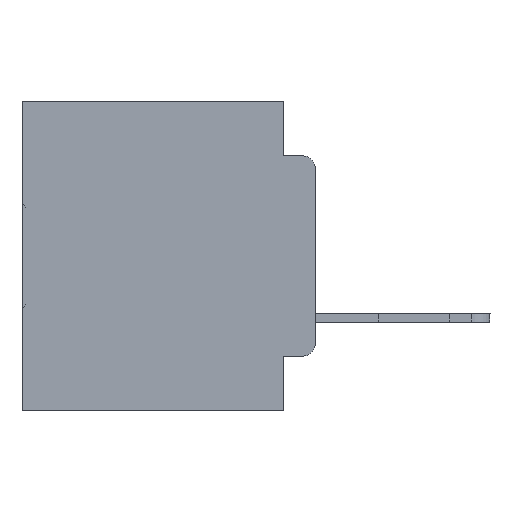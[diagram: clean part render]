
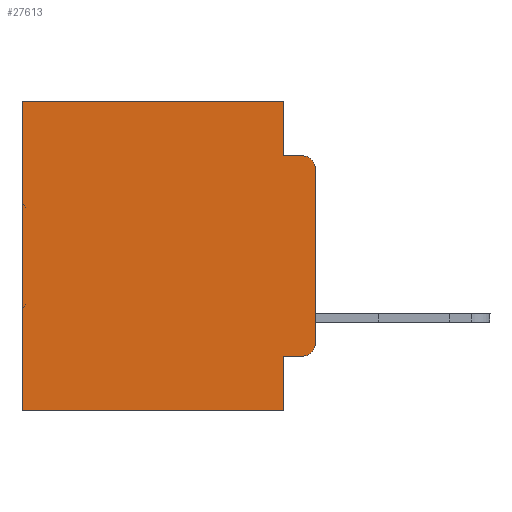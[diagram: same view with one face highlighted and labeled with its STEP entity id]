
A CAD part, left-side view. The second image highlights one B-rep face of the part: STEP entity #27613.
In plain terms, the highlighted planar face has unit normal (-1, 0, 0).
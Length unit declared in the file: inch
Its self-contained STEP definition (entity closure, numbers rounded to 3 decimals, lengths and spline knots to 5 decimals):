
#480 = LINE ( 'NONE', #10816, #10566 ) ;
#767 = EDGE_CURVE ( 'NONE', #8876, #31072, #8482, .T. ) ;
#923 = DIRECTION ( 'NONE',  ( -1., 0., 0. ) ) ;
#1923 = EDGE_CURVE ( 'NONE', #31454, #28247, #25120, .T. ) ;
#2304 = AXIS2_PLACEMENT_3D ( 'NONE', #2884, #13237, #32821 ) ;
#2442 = EDGE_CURVE ( 'NONE', #24486, #17753, #480, .T. ) ;
#2659 = AXIS2_PLACEMENT_3D ( 'NONE', #26231, #3003, #18583 ) ;
#2714 = CARTESIAN_POINT ( 'NONE',  ( 0.298, 0., -0.1085 ) ) ;
#2884 = CARTESIAN_POINT ( 'NONE',  ( 0.298, 0.02, -0.3915 ) ) ;
#3003 = DIRECTION ( 'NONE',  ( 1., 0., 0. ) ) ;
#3346 = DIRECTION ( 'NONE',  ( 0., 1., 0. ) ) ;
#4257 = CARTESIAN_POINT ( 'NONE',  ( 0.298, 0.051, -0.0885 ) ) ;
#4644 = LINE ( 'NONE', #18010, #33050 ) ;
#4717 = LINE ( 'NONE', #33357, #30166 ) ;
#4857 = ORIENTED_EDGE ( 'NONE', *, *, #19852, .F. ) ;
#5073 = ORIENTED_EDGE ( 'NONE', *, *, #25965, .T. ) ;
#5228 = CARTESIAN_POINT ( 'NONE',  ( 0.298, 0.02, -0.4115 ) ) ;
#5541 = PLANE ( 'NONE',  #2659 ) ;
#5566 = VERTEX_POINT ( 'NONE', #30601 ) ;
#6061 = VECTOR ( 'NONE', #18292, 39.37008 ) ;
#6773 = VECTOR ( 'NONE', #13849, 39.37008 ) ;
#7393 = ORIENTED_EDGE ( 'NONE', *, *, #12157, .T. ) ;
#8482 = LINE ( 'NONE', #10684, #6061 ) ;
#8688 = CARTESIAN_POINT ( 'NONE',  ( 0.298, 0.473, -0.5 ) ) ;
#8876 = VERTEX_POINT ( 'NONE', #24461 ) ;
#9707 = DIRECTION ( 'NONE',  ( 0., 0., -1. ) ) ;
#10122 = CARTESIAN_POINT ( 'NONE',  ( 0.298, 0.051, -0.4115 ) ) ;
#10221 = ORIENTED_EDGE ( 'NONE', *, *, #15352, .T. ) ;
#10566 = VECTOR ( 'NONE', #3346, 39.37008 ) ;
#10684 = CARTESIAN_POINT ( 'NONE',  ( 0.298, 0.051, 0. ) ) ;
#10816 = CARTESIAN_POINT ( 'NONE',  ( 0.298, 0., -0.5 ) ) ;
#10914 = VERTEX_POINT ( 'NONE', #5228 ) ;
#11928 = VERTEX_POINT ( 'NONE', #33470 ) ;
#12157 = EDGE_CURVE ( 'NONE', #11928, #17753, #19893, .T. ) ;
#12678 = DIRECTION ( 'NONE',  ( 0., -1., 0. ) ) ;
#12730 = EDGE_LOOP ( 'NONE', ( #21967, #5073, #28135, #15544, #18105, #7393, #22763, #4857, #10221, #15747 ) ) ;
#13237 = DIRECTION ( 'NONE',  ( -1., 0., 0. ) ) ;
#13849 = DIRECTION ( 'NONE',  ( 0., 1., 0. ) ) ;
#14605 = LINE ( 'NONE', #4257, #22211 ) ;
#15277 = CARTESIAN_POINT ( 'NONE',  ( 0.298, 0., 0. ) ) ;
#15352 = EDGE_CURVE ( 'NONE', #32361, #10914, #4717, .T. ) ;
#15539 = AXIS2_PLACEMENT_3D ( 'NONE', #24161, #923, #21758 ) ;
#15544 = ORIENTED_EDGE ( 'NONE', *, *, #767, .F. ) ;
#15747 = ORIENTED_EDGE ( 'NONE', *, *, #20440, .T. ) ;
#16549 = CARTESIAN_POINT ( 'NONE',  ( 0.298, 0., 0. ) ) ;
#17753 = VERTEX_POINT ( 'NONE', #8688 ) ;
#17786 = EDGE_CURVE ( 'NONE', #31072, #5566, #14605, .T. ) ;
#18010 = CARTESIAN_POINT ( 'NONE',  ( 0.298, 0.051, 0. ) ) ;
#18105 = ORIENTED_EDGE ( 'NONE', *, *, #24098, .T. ) ;
#18292 = DIRECTION ( 'NONE',  ( 0., 0., -1. ) ) ;
#18414 = FACE_OUTER_BOUND ( 'NONE', #12730, .T. ) ;
#18583 = DIRECTION ( 'NONE',  ( 0., 0., -1. ) ) ;
#19852 = EDGE_CURVE ( 'NONE', #32361, #24486, #4644, .T. ) ;
#19893 = LINE ( 'NONE', #30205, #21431 ) ;
#20440 = EDGE_CURVE ( 'NONE', #10914, #28247, #26115, .T. ) ;
#20728 = DIRECTION ( 'NONE',  ( 0., 0., -1. ) ) ;
#21331 = VECTOR ( 'NONE', #9707, 39.37008 ) ;
#21431 = VECTOR ( 'NONE', #27514, 39.37008 ) ;
#21758 = DIRECTION ( 'NONE',  ( 0., 0., -1. ) ) ;
#21798 = LINE ( 'NONE', #16549, #6773 ) ;
#21967 = ORIENTED_EDGE ( 'NONE', *, *, #1923, .F. ) ;
#22211 = VECTOR ( 'NONE', #27152, 39.37008 ) ;
#22763 = ORIENTED_EDGE ( 'NONE', *, *, #2442, .F. ) ;
#23158 = CIRCLE ( 'NONE', #15539, 0.02 ) ;
#24098 = EDGE_CURVE ( 'NONE', #8876, #11928, #21798, .T. ) ;
#24161 = CARTESIAN_POINT ( 'NONE',  ( 0.298, 0.02, -0.1085 ) ) ;
#24182 = CARTESIAN_POINT ( 'NONE',  ( 0.298, 0.051, -0.0885 ) ) ;
#24461 = CARTESIAN_POINT ( 'NONE',  ( 0.298, 0.051, 0. ) ) ;
#24486 = VERTEX_POINT ( 'NONE', #26017 ) ;
#25120 = LINE ( 'NONE', #15277, #21331 ) ;
#25965 = EDGE_CURVE ( 'NONE', #31454, #5566, #23158, .T. ) ;
#26017 = CARTESIAN_POINT ( 'NONE',  ( 0.298, 0.051, -0.5 ) ) ;
#26115 = CIRCLE ( 'NONE', #2304, 0.02 ) ;
#26231 = CARTESIAN_POINT ( 'NONE',  ( 0.298, 0., 0. ) ) ;
#27152 = DIRECTION ( 'NONE',  ( 0., -1., 0. ) ) ;
#27514 = DIRECTION ( 'NONE',  ( 0., 0., -1. ) ) ;
#27613 = ADVANCED_FACE ( 'NONE', ( #18414 ), #5541, .F. ) ;
#28135 = ORIENTED_EDGE ( 'NONE', *, *, #17786, .F. ) ;
#28247 = VERTEX_POINT ( 'NONE', #29563 ) ;
#29563 = CARTESIAN_POINT ( 'NONE',  ( 0.298, 0., -0.3915 ) ) ;
#30166 = VECTOR ( 'NONE', #12678, 39.37008 ) ;
#30205 = CARTESIAN_POINT ( 'NONE',  ( 0.298, 0.473, 0. ) ) ;
#30601 = CARTESIAN_POINT ( 'NONE',  ( 0.298, 0.02, -0.0885 ) ) ;
#31072 = VERTEX_POINT ( 'NONE', #24182 ) ;
#31454 = VERTEX_POINT ( 'NONE', #2714 ) ;
#32361 = VERTEX_POINT ( 'NONE', #10122 ) ;
#32821 = DIRECTION ( 'NONE',  ( 0., 0., -1. ) ) ;
#33050 = VECTOR ( 'NONE', #20728, 39.37008 ) ;
#33357 = CARTESIAN_POINT ( 'NONE',  ( 0.298, 0.051, -0.4115 ) ) ;
#33470 = CARTESIAN_POINT ( 'NONE',  ( 0.298, 0.473, 0. ) ) ;
